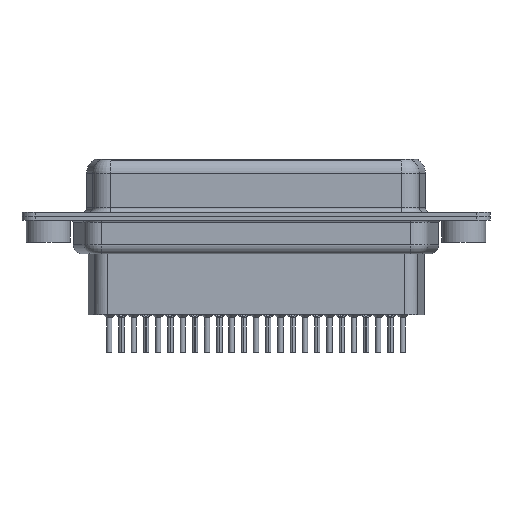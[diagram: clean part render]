
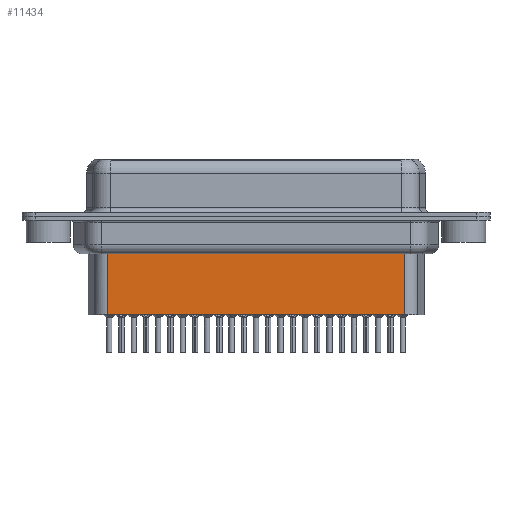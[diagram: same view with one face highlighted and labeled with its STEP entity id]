
A CAD part, front view. The second image highlights one B-rep face of the part: STEP entity #11434.
In plain terms, the highlighted planar face has unit normal (0, -1, 0).
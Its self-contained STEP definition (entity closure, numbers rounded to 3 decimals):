
#69 = LINE ( 'NONE', #6327, #8257 ) ;
#1378 = VECTOR ( 'NONE', #27246, 1000. ) ;
#1437 = DIRECTION ( 'NONE',  ( 1., 0., 0. ) ) ;
#3496 = LINE ( 'NONE', #14508, #8020 ) ;
#4144 = VERTEX_POINT ( 'NONE', #8212 ) ;
#4646 = ORIENTED_EDGE ( 'NONE', *, *, #5108, .T. ) ;
#5108 = EDGE_CURVE ( 'NONE', #9564, #7893, #3496, .T. ) ;
#5180 = ORIENTED_EDGE ( 'NONE', *, *, #18843, .T. ) ;
#5425 = ORIENTED_EDGE ( 'NONE', *, *, #10534, .F. ) ;
#6327 = CARTESIAN_POINT ( 'NONE',  ( 6.706, -3.5, -11.15 ) ) ;
#6407 = LINE ( 'NONE', #8788, #14372 ) ;
#6681 = DIRECTION ( 'NONE',  ( 0., 0., -1. ) ) ;
#7893 = VERTEX_POINT ( 'NONE', #27913 ) ;
#8020 = VECTOR ( 'NONE', #23086, 1000. ) ;
#8212 = CARTESIAN_POINT ( 'NONE',  ( 40.344, -3.5, -11.15 ) ) ;
#8257 = VECTOR ( 'NONE', #14802, 1000. ) ;
#8324 = CARTESIAN_POINT ( 'NONE',  ( 40.344, -3.5, -4.097 ) ) ;
#8788 = CARTESIAN_POINT ( 'NONE',  ( 40.344, -3.5, -3.1 ) ) ;
#9132 = EDGE_LOOP ( 'NONE', ( #5425, #5180, #4646, #15358 ) ) ;
#9564 = VERTEX_POINT ( 'NONE', #11994 ) ;
#10058 = LINE ( 'NONE', #16688, #1378 ) ;
#10534 = EDGE_CURVE ( 'NONE', #19372, #4144, #6407, .T. ) ;
#11434 = ADVANCED_FACE ( 'NONE', ( #27379 ), #27243, .T. ) ;
#11994 = CARTESIAN_POINT ( 'NONE',  ( 6.706, -3.5, -4.097 ) ) ;
#12195 = DIRECTION ( 'NONE',  ( 0., -1., 0. ) ) ;
#14372 = VECTOR ( 'NONE', #6681, 1000. ) ;
#14508 = CARTESIAN_POINT ( 'NONE',  ( 6.706, -3.5, -3.1 ) ) ;
#14802 = DIRECTION ( 'NONE',  ( -1., 0., 0. ) ) ;
#15358 = ORIENTED_EDGE ( 'NONE', *, *, #16336, .F. ) ;
#16336 = EDGE_CURVE ( 'NONE', #4144, #7893, #69, .T. ) ;
#16646 = AXIS2_PLACEMENT_3D ( 'NONE', #21177, #12195, #1437 ) ;
#16688 = CARTESIAN_POINT ( 'NONE',  ( 6.459, -3.5, -4.097 ) ) ;
#18843 = EDGE_CURVE ( 'NONE', #19372, #9564, #10058, .T. ) ;
#19372 = VERTEX_POINT ( 'NONE', #8324 ) ;
#21177 = CARTESIAN_POINT ( 'NONE',  ( 6.706, -3.5, -3.1 ) ) ;
#23086 = DIRECTION ( 'NONE',  ( 0., 0., -1. ) ) ;
#27243 = PLANE ( 'NONE',  #16646 ) ;
#27246 = DIRECTION ( 'NONE',  ( -1., 0., 0. ) ) ;
#27379 = FACE_OUTER_BOUND ( 'NONE', #9132, .T. ) ;
#27913 = CARTESIAN_POINT ( 'NONE',  ( 6.706, -3.5, -11.15 ) ) ;
